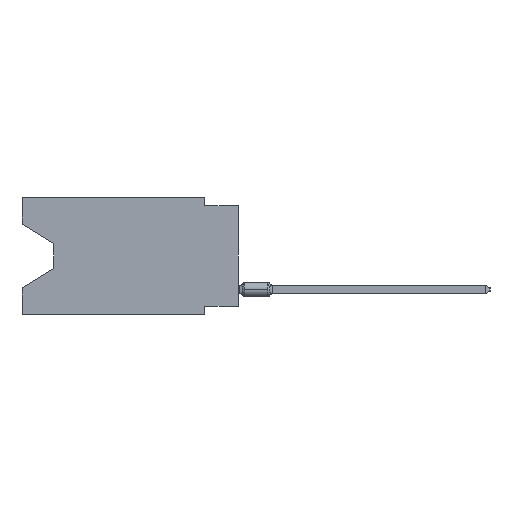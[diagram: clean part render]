
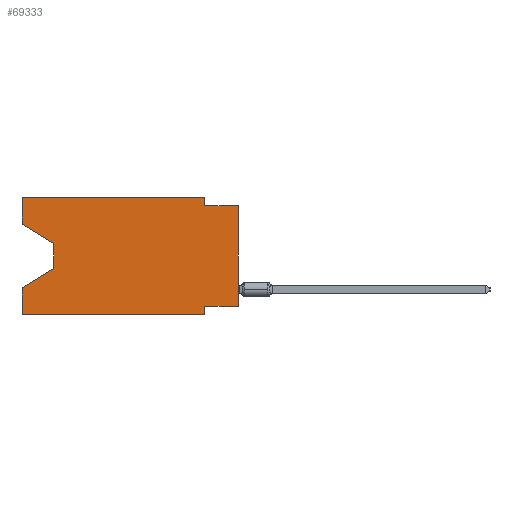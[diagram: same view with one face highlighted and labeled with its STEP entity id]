
A CAD part, left-side view. The second image highlights one B-rep face of the part: STEP entity #69333.
In plain terms, the highlighted planar face has unit normal (-1, 0, 0).
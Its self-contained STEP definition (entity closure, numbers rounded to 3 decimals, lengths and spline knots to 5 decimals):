
#75 = VERTEX_POINT ( 'NONE', #13660 ) ;
#161 = LINE ( 'NONE', #60924, #110000 ) ;
#1133 = CARTESIAN_POINT ( 'NONE',  ( 0., 0.645, -0.08025 ) ) ;
#3842 = DIRECTION ( 'NONE',  ( 1., 0., 0. ) ) ;
#4899 = EDGE_CURVE ( 'NONE', #80729, #20058, #24889, .T. ) ;
#9561 = VECTOR ( 'NONE', #23503, 39.37008 ) ;
#10282 = DIRECTION ( 'NONE',  ( 0., 0., -1. ) ) ;
#11851 = EDGE_CURVE ( 'NONE', #32005, #95415, #161, .T. ) ;
#11960 = EDGE_CURVE ( 'NONE', #80729, #99671, #62031, .T. ) ;
#12477 = VECTOR ( 'NONE', #106214, 39.37008 ) ;
#12855 = VECTOR ( 'NONE', #30851, 39.37008 ) ;
#13660 = CARTESIAN_POINT ( 'NONE',  ( 0., 0.55, -0.212 ) ) ;
#16806 = DIRECTION ( 'NONE',  ( 0., 1., 0. ) ) ;
#19635 = EDGE_CURVE ( 'NONE', #95415, #88831, #42094, .T. ) ;
#19648 = DIRECTION ( 'NONE',  ( 0., -1., 0. ) ) ;
#20058 = VERTEX_POINT ( 'NONE', #77080 ) ;
#20897 = VECTOR ( 'NONE', #16806, 39.37008 ) ;
#23389 = VECTOR ( 'NONE', #10282, 39.37008 ) ;
#23503 = DIRECTION ( 'NONE',  ( 0., 0., 1. ) ) ;
#24889 = LINE ( 'NONE', #85630, #69758 ) ;
#25745 = CARTESIAN_POINT ( 'NONE',  ( 0., 0.645, -0.35 ) ) ;
#26457 = VERTEX_POINT ( 'NONE', #44485 ) ;
#26616 = ORIENTED_EDGE ( 'NONE', *, *, #59368, .T. ) ;
#27835 = DIRECTION ( 'NONE',  ( 0., 0., -1. ) ) ;
#28273 = LINE ( 'NONE', #36646, #71479 ) ;
#29338 = LINE ( 'NONE', #87890, #42850 ) ;
#30176 = LINE ( 'NONE', #107661, #105516 ) ;
#30390 = CARTESIAN_POINT ( 'NONE',  ( 0., 0.55, -0.138 ) ) ;
#30471 = CARTESIAN_POINT ( 'NONE',  ( 0., 0.1, -0.025 ) ) ;
#30851 = DIRECTION ( 'NONE',  ( 0., -0.855, -0.519 ) ) ;
#31903 = LINE ( 'NONE', #65897, #9561 ) ;
#32005 = VERTEX_POINT ( 'NONE', #83102 ) ;
#36646 = CARTESIAN_POINT ( 'NONE',  ( 0., 0.55, -0.212 ) ) ;
#37174 = DIRECTION ( 'NONE',  ( 0., 0., -1. ) ) ;
#38187 = AXIS2_PLACEMENT_3D ( 'NONE', #71881, #3842, #27835 ) ;
#39225 = CARTESIAN_POINT ( 'NONE',  ( 0., 0.645, -0.08025 ) ) ;
#40298 = EDGE_LOOP ( 'NONE', ( #53073, #26616, #53766, #72014, #79098, #107968, #90022, #99368, #99541, #73241, #82171, #81912 ) ) ;
#41911 = CARTESIAN_POINT ( 'NONE',  ( 0., 0., -0.325 ) ) ;
#42094 = LINE ( 'NONE', #86100, #23389 ) ;
#42850 = VECTOR ( 'NONE', #37174, 39.37008 ) ;
#44485 = CARTESIAN_POINT ( 'NONE',  ( 0., 0., -0.325 ) ) ;
#46101 = CARTESIAN_POINT ( 'NONE',  ( 0., 0., -0.025 ) ) ;
#46128 = DIRECTION ( 'NONE',  ( 0., 0.855, -0.519 ) ) ;
#47948 = EDGE_CURVE ( 'NONE', #50429, #32005, #31903, .T. ) ;
#50429 = VERTEX_POINT ( 'NONE', #1133 ) ;
#53073 = ORIENTED_EDGE ( 'NONE', *, *, #90119, .T. ) ;
#53398 = EDGE_CURVE ( 'NONE', #105448, #99671, #29338, .T. ) ;
#53766 = ORIENTED_EDGE ( 'NONE', *, *, #87249, .T. ) ;
#55335 = CARTESIAN_POINT ( 'NONE',  ( 0., 0.645, -0.35 ) ) ;
#56385 = DIRECTION ( 'NONE',  ( 0., -1., 0. ) ) ;
#59368 = EDGE_CURVE ( 'NONE', #80463, #75, #107869, .T. ) ;
#60476 = LINE ( 'NONE', #102830, #95725 ) ;
#60924 = CARTESIAN_POINT ( 'NONE',  ( 0., 0.645, 0. ) ) ;
#62031 = LINE ( 'NONE', #55335, #63700 ) ;
#63700 = VECTOR ( 'NONE', #19648, 39.37008 ) ;
#64411 = CARTESIAN_POINT ( 'NONE',  ( 0., 0.1, -0.325 ) ) ;
#64876 = LINE ( 'NONE', #39225, #12855 ) ;
#65897 = CARTESIAN_POINT ( 'NONE',  ( 0., 0.645, 0. ) ) ;
#69333 = ADVANCED_FACE ( 'NONE', ( #96409 ), #89150, .F. ) ;
#69758 = VECTOR ( 'NONE', #100725, 39.37008 ) ;
#71479 = VECTOR ( 'NONE', #46128, 39.37008 ) ;
#71881 = CARTESIAN_POINT ( 'NONE',  ( 0., 0.645, 0. ) ) ;
#72014 = ORIENTED_EDGE ( 'NONE', *, *, #4899, .F. ) ;
#72572 = CARTESIAN_POINT ( 'NONE',  ( 0., 0.1, 0. ) ) ;
#73241 = ORIENTED_EDGE ( 'NONE', *, *, #19635, .F. ) ;
#77080 = CARTESIAN_POINT ( 'NONE',  ( 0., 0.645, -0.26975 ) ) ;
#79098 = ORIENTED_EDGE ( 'NONE', *, *, #11960, .T. ) ;
#80463 = VERTEX_POINT ( 'NONE', #97205 ) ;
#80729 = VERTEX_POINT ( 'NONE', #25745 ) ;
#81912 = ORIENTED_EDGE ( 'NONE', *, *, #47948, .F. ) ;
#82171 = ORIENTED_EDGE ( 'NONE', *, *, #11851, .F. ) ;
#82990 = VERTEX_POINT ( 'NONE', #46101 ) ;
#83102 = CARTESIAN_POINT ( 'NONE',  ( 0., 0.645, 0. ) ) ;
#84558 = CARTESIAN_POINT ( 'NONE',  ( 0., 0.1, -0.35 ) ) ;
#85630 = CARTESIAN_POINT ( 'NONE',  ( 0., 0.645, 0. ) ) ;
#85930 = EDGE_CURVE ( 'NONE', #26457, #82990, #60476, .T. ) ;
#86100 = CARTESIAN_POINT ( 'NONE',  ( 0., 0.1, 0. ) ) ;
#87249 = EDGE_CURVE ( 'NONE', #75, #20058, #28273, .T. ) ;
#87890 = CARTESIAN_POINT ( 'NONE',  ( 0., 0.1, -0.35 ) ) ;
#88831 = VERTEX_POINT ( 'NONE', #30471 ) ;
#89150 = PLANE ( 'NONE',  #38187 ) ;
#90022 = ORIENTED_EDGE ( 'NONE', *, *, #108260, .F. ) ;
#90119 = EDGE_CURVE ( 'NONE', #50429, #80463, #64876, .T. ) ;
#90592 = EDGE_CURVE ( 'NONE', #88831, #82990, #30176, .T. ) ;
#93169 = LINE ( 'NONE', #41911, #20897 ) ;
#94912 = DIRECTION ( 'NONE',  ( 0., -1., 0. ) ) ;
#95012 = DIRECTION ( 'NONE',  ( 0., 0., 1. ) ) ;
#95415 = VERTEX_POINT ( 'NONE', #72572 ) ;
#95725 = VECTOR ( 'NONE', #95012, 39.37008 ) ;
#96409 = FACE_OUTER_BOUND ( 'NONE', #40298, .T. ) ;
#97205 = CARTESIAN_POINT ( 'NONE',  ( 0., 0.55, -0.138 ) ) ;
#99368 = ORIENTED_EDGE ( 'NONE', *, *, #85930, .T. ) ;
#99541 = ORIENTED_EDGE ( 'NONE', *, *, #90592, .F. ) ;
#99671 = VERTEX_POINT ( 'NONE', #84558 ) ;
#100725 = DIRECTION ( 'NONE',  ( 0., 0., 1. ) ) ;
#102830 = CARTESIAN_POINT ( 'NONE',  ( 0., 0., 0. ) ) ;
#105448 = VERTEX_POINT ( 'NONE', #64411 ) ;
#105516 = VECTOR ( 'NONE', #56385, 39.37008 ) ;
#106214 = DIRECTION ( 'NONE',  ( 0., 0., -1. ) ) ;
#107661 = CARTESIAN_POINT ( 'NONE',  ( 0., 0., -0.025 ) ) ;
#107869 = LINE ( 'NONE', #30390, #12477 ) ;
#107968 = ORIENTED_EDGE ( 'NONE', *, *, #53398, .F. ) ;
#108260 = EDGE_CURVE ( 'NONE', #26457, #105448, #93169, .T. ) ;
#110000 = VECTOR ( 'NONE', #94912, 39.37008 ) ;
